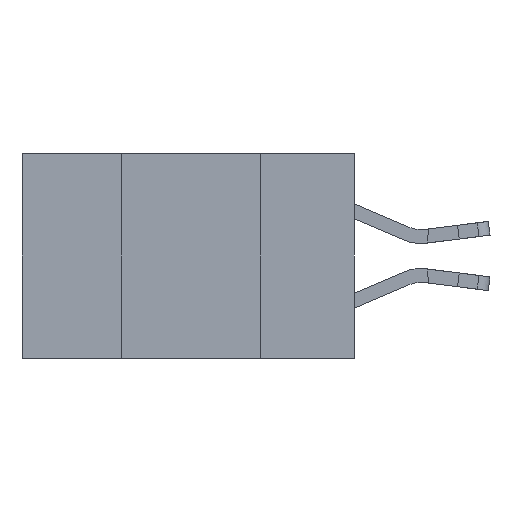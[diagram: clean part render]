
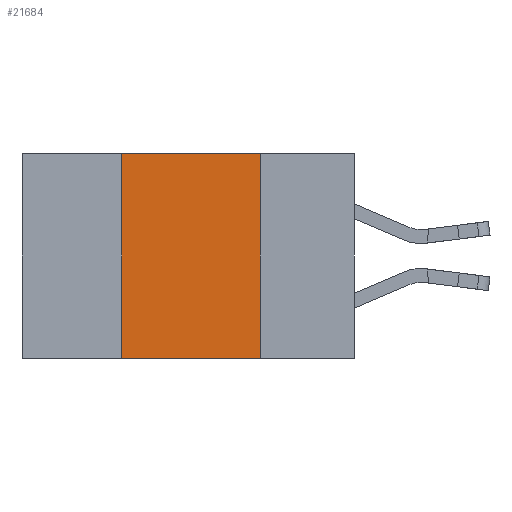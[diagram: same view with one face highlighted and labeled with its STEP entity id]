
A CAD part, left-side view. The second image highlights one B-rep face of the part: STEP entity #21684.
In plain terms, the highlighted planar face has unit normal (-1, 0, 0).
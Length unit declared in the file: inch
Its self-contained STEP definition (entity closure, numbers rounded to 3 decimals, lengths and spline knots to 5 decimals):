
#161 = CARTESIAN_POINT ( 'NONE',  ( 0., 0.17, -0.37 ) ) ;
#191 = CARTESIAN_POINT ( 'NONE',  ( 0., 0.42, 0. ) ) ;
#607 = CARTESIAN_POINT ( 'NONE',  ( 0., 0.42, -0.37 ) ) ;
#2151 = LINE ( 'NONE', #23695, #21796 ) ;
#2962 = EDGE_CURVE ( 'NONE', #14403, #20012, #3118, .T. ) ;
#3118 = LINE ( 'NONE', #8476, #22712 ) ;
#3493 = AXIS2_PLACEMENT_3D ( 'NONE', #21400, #8391, #21476 ) ;
#3655 = ORIENTED_EDGE ( 'NONE', *, *, #2962, .T. ) ;
#3974 = EDGE_LOOP ( 'NONE', ( #22040, #7672, #13231, #3655 ) ) ;
#4098 = DIRECTION ( 'NONE',  ( 0., -1., 0. ) ) ;
#4295 = EDGE_CURVE ( 'NONE', #14403, #16087, #2151, .T. ) ;
#4366 = VECTOR ( 'NONE', #4098, 39.37008 ) ;
#4991 = EDGE_CURVE ( 'NONE', #14427, #20012, #12095, .T. ) ;
#7672 = ORIENTED_EDGE ( 'NONE', *, *, #13186, .F. ) ;
#8112 = DIRECTION ( 'NONE',  ( 0., -1., 0. ) ) ;
#8391 = DIRECTION ( 'NONE',  ( 1., 0., 0. ) ) ;
#8476 = CARTESIAN_POINT ( 'NONE',  ( 0., 0.6, -0.37 ) ) ;
#9558 = DIRECTION ( 'NONE',  ( 0., 0., 1. ) ) ;
#9579 = LINE ( 'NONE', #17357, #4366 ) ;
#11538 = VECTOR ( 'NONE', #23612, 39.37008 ) ;
#12095 = LINE ( 'NONE', #22476, #11538 ) ;
#13186 = EDGE_CURVE ( 'NONE', #16087, #14427, #9579, .T. ) ;
#13231 = ORIENTED_EDGE ( 'NONE', *, *, #4295, .F. ) ;
#14403 = VERTEX_POINT ( 'NONE', #607 ) ;
#14427 = VERTEX_POINT ( 'NONE', #15876 ) ;
#15876 = CARTESIAN_POINT ( 'NONE',  ( 0., 0.17, 0. ) ) ;
#16087 = VERTEX_POINT ( 'NONE', #191 ) ;
#17357 = CARTESIAN_POINT ( 'NONE',  ( 0., 0.6, 0. ) ) ;
#17502 = FACE_OUTER_BOUND ( 'NONE', #3974, .T. ) ;
#19609 = PLANE ( 'NONE',  #3493 ) ;
#20012 = VERTEX_POINT ( 'NONE', #161 ) ;
#21400 = CARTESIAN_POINT ( 'NONE',  ( 0., 0.6, 0. ) ) ;
#21476 = DIRECTION ( 'NONE',  ( 0., 0., -1. ) ) ;
#21684 = ADVANCED_FACE ( 'NONE', ( #17502 ), #19609, .F. ) ;
#21796 = VECTOR ( 'NONE', #9558, 39.37008 ) ;
#22040 = ORIENTED_EDGE ( 'NONE', *, *, #4991, .F. ) ;
#22476 = CARTESIAN_POINT ( 'NONE',  ( 0., 0.17, 0. ) ) ;
#22712 = VECTOR ( 'NONE', #8112, 39.37008 ) ;
#23612 = DIRECTION ( 'NONE',  ( 0., 0., -1. ) ) ;
#23695 = CARTESIAN_POINT ( 'NONE',  ( 0., 0.42, 0. ) ) ;
